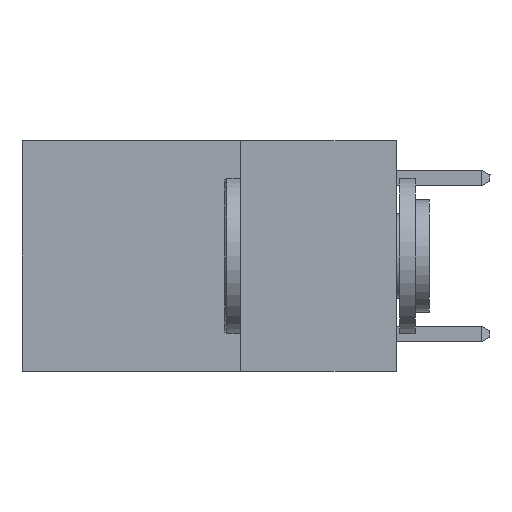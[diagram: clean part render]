
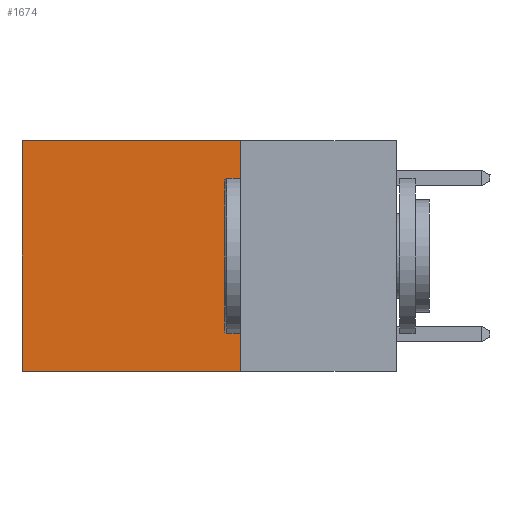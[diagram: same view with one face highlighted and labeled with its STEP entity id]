
A CAD part, left-side view. The second image highlights one B-rep face of the part: STEP entity #1674.
In plain terms, the highlighted planar face has unit normal (-1, 0, 0).
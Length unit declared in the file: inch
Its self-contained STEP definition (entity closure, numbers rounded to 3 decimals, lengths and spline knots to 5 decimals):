
#1223 = CARTESIAN_POINT ( 'NONE',  ( 0.2625, 0.6, 0. ) ) ;
#1475 = EDGE_CURVE ( 'NONE', #10983, #6892, #12437, .T. ) ;
#1674 = ADVANCED_FACE ( 'NONE', ( #17666 ), #8802, .F. ) ;
#1913 = ORIENTED_EDGE ( 'NONE', *, *, #14931, .F. ) ;
#2412 = VECTOR ( 'NONE', #5031, 39.37008 ) ;
#2834 = CARTESIAN_POINT ( 'NONE',  ( 0.2625, 0.25, -0.37 ) ) ;
#3295 = EDGE_CURVE ( 'NONE', #6892, #18622, #11427, .T. ) ;
#3971 = VERTEX_POINT ( 'NONE', #2834 ) ;
#4340 = CARTESIAN_POINT ( 'NONE',  ( 0.2625, 0.25, 0. ) ) ;
#5031 = DIRECTION ( 'NONE',  ( 0., 1., 0. ) ) ;
#5423 = VECTOR ( 'NONE', #6459, 39.37008 ) ;
#5684 = CARTESIAN_POINT ( 'NONE',  ( 0.2625, 0.25, 0. ) ) ;
#6013 = VECTOR ( 'NONE', #7139, 39.37008 ) ;
#6459 = DIRECTION ( 'NONE',  ( 0., 1., 0. ) ) ;
#6848 = CARTESIAN_POINT ( 'NONE',  ( 0.2625, 0.6, 0. ) ) ;
#6892 = VERTEX_POINT ( 'NONE', #1223 ) ;
#7139 = DIRECTION ( 'NONE',  ( 0., 0., -1. ) ) ;
#7351 = AXIS2_PLACEMENT_3D ( 'NONE', #4340, #18057, #10562 ) ;
#8234 = CARTESIAN_POINT ( 'NONE',  ( 0.2625, 0.25, 0. ) ) ;
#8638 = EDGE_CURVE ( 'NONE', #10983, #3971, #13120, .T. ) ;
#8802 = PLANE ( 'NONE',  #7351 ) ;
#9201 = ORIENTED_EDGE ( 'NONE', *, *, #3295, .T. ) ;
#10562 = DIRECTION ( 'NONE',  ( 0., 0., -1. ) ) ;
#10983 = VERTEX_POINT ( 'NONE', #5684 ) ;
#11427 = LINE ( 'NONE', #6848, #6013 ) ;
#11962 = EDGE_LOOP ( 'NONE', ( #9201, #1913, #16125, #12361 ) ) ;
#12361 = ORIENTED_EDGE ( 'NONE', *, *, #1475, .T. ) ;
#12387 = CARTESIAN_POINT ( 'NONE',  ( 0.2625, 0.6, -0.37 ) ) ;
#12437 = LINE ( 'NONE', #8234, #2412 ) ;
#13120 = LINE ( 'NONE', #16047, #18718 ) ;
#14931 = EDGE_CURVE ( 'NONE', #3971, #18622, #15313, .T. ) ;
#15313 = LINE ( 'NONE', #18333, #5423 ) ;
#15766 = DIRECTION ( 'NONE',  ( 0., 0., -1. ) ) ;
#16047 = CARTESIAN_POINT ( 'NONE',  ( 0.2625, 0.25, 0. ) ) ;
#16125 = ORIENTED_EDGE ( 'NONE', *, *, #8638, .F. ) ;
#17666 = FACE_OUTER_BOUND ( 'NONE', #11962, .T. ) ;
#18057 = DIRECTION ( 'NONE',  ( 1., 0., 0. ) ) ;
#18333 = CARTESIAN_POINT ( 'NONE',  ( 0.2625, 0.25, -0.37 ) ) ;
#18622 = VERTEX_POINT ( 'NONE', #12387 ) ;
#18718 = VECTOR ( 'NONE', #15766, 39.37008 ) ;
